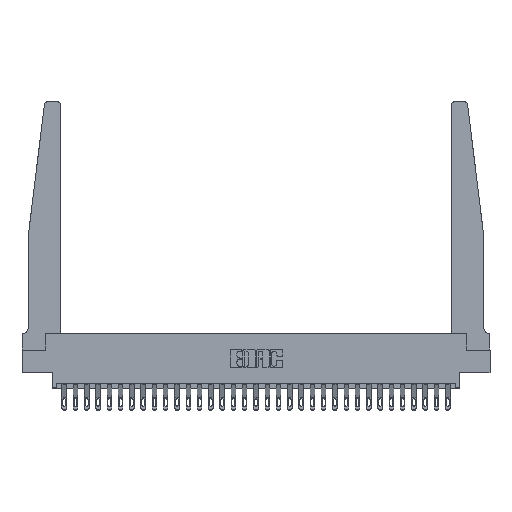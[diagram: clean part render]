
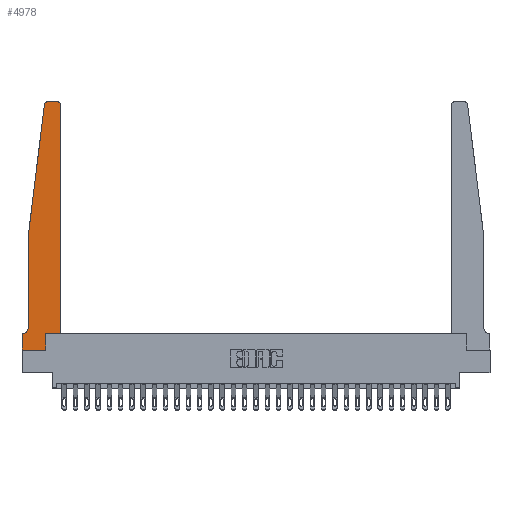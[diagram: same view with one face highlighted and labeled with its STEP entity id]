
A CAD part, top view. The second image highlights one B-rep face of the part: STEP entity #4978.
In plain terms, the highlighted planar face has unit normal (0, 0, 1).
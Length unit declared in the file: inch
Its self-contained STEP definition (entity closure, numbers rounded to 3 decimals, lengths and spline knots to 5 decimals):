
#320 = DIRECTION ( 'NONE',  ( 1., 0., 0. ) ) ;
#782 = VECTOR ( 'NONE', #8083, 39.37008 ) ;
#801 = VECTOR ( 'NONE', #20640, 39.37008 ) ;
#812 = CARTESIAN_POINT ( 'NONE',  ( 0.425, 0.18, 0.37 ) ) ;
#824 = AXIS2_PLACEMENT_3D ( 'NONE', #27190, #13727, #320 ) ;
#2477 = EDGE_CURVE ( 'NONE', #11949, #20682, #16619, .T. ) ;
#2863 = VERTEX_POINT ( 'NONE', #5621 ) ;
#3533 = CARTESIAN_POINT ( 'NONE',  ( 0.27653, 2.75, 0.37 ) ) ;
#3816 = EDGE_CURVE ( 'NONE', #6763, #6509, #17950, .T. ) ;
#3834 = VERTEX_POINT ( 'NONE', #5070 ) ;
#4319 = CARTESIAN_POINT ( 'NONE',  ( 0.2605, 0., 0.37 ) ) ;
#4370 = CARTESIAN_POINT ( 'NONE',  ( 0.395, 2.75, 0.37 ) ) ;
#4636 = DIRECTION ( 'NONE',  ( 0., 0., -1. ) ) ;
#4846 = CARTESIAN_POINT ( 'NONE',  ( 0., 0.1875, 0.37 ) ) ;
#4978 = ADVANCED_FACE ( 'NONE', ( #24131 ), #9467, .T. ) ;
#5057 = EDGE_CURVE ( 'NONE', #20908, #8378, #22018, .T. ) ;
#5070 = CARTESIAN_POINT ( 'NONE',  ( 0.015, 0.1875, 0.37 ) ) ;
#5209 = CIRCLE ( 'NONE', #824, 0.03 ) ;
#5621 = CARTESIAN_POINT ( 'NONE',  ( 0.425, 0.18, 0.37 ) ) ;
#6509 = VERTEX_POINT ( 'NONE', #3533 ) ;
#6750 = LINE ( 'NONE', #12464, #782 ) ;
#6763 = VERTEX_POINT ( 'NONE', #4370 ) ;
#7297 = ORIENTED_EDGE ( 'NONE', *, *, #3816, .T. ) ;
#7327 = DIRECTION ( 'NONE',  ( 1., 0., 0. ) ) ;
#7530 = CARTESIAN_POINT ( 'NONE',  ( 0., 0., 0.37 ) ) ;
#7535 = DIRECTION ( 'NONE',  ( 0., -1., 0. ) ) ;
#7594 = ORIENTED_EDGE ( 'NONE', *, *, #27460, .T. ) ;
#7862 = VERTEX_POINT ( 'NONE', #24970 ) ;
#7977 = VECTOR ( 'NONE', #26156, 39.37008 ) ;
#8083 = DIRECTION ( 'NONE',  ( -0.122, -0.992, 0. ) ) ;
#8378 = VERTEX_POINT ( 'NONE', #18049 ) ;
#8892 = ORIENTED_EDGE ( 'NONE', *, *, #24839, .T. ) ;
#9230 = ORIENTED_EDGE ( 'NONE', *, *, #19029, .T. ) ;
#9361 = VECTOR ( 'NONE', #14224, 39.37008 ) ;
#9467 = PLANE ( 'NONE',  #29012 ) ;
#10032 = CARTESIAN_POINT ( 'NONE',  ( 0.2605, 0.18, 0.37 ) ) ;
#10102 = VECTOR ( 'NONE', #7535, 39.37008 ) ;
#10426 = CARTESIAN_POINT ( 'NONE',  ( 0.395, 2.72, 0.37 ) ) ;
#10436 = CARTESIAN_POINT ( 'NONE',  ( 0., 0., 0.37 ) ) ;
#10691 = VECTOR ( 'NONE', #20111, 39.37008 ) ;
#10889 = CARTESIAN_POINT ( 'NONE',  ( 0.065, 1.25, 0.37 ) ) ;
#11316 = EDGE_CURVE ( 'NONE', #8378, #3834, #21455, .T. ) ;
#11502 = AXIS2_PLACEMENT_3D ( 'NONE', #10426, #26145, #12683 ) ;
#11662 = LINE ( 'NONE', #11758, #28841 ) ;
#11714 = DIRECTION ( 'NONE',  ( 0., 0., 1. ) ) ;
#11734 = CARTESIAN_POINT ( 'NONE',  ( 0.25, 2.75, 0.37 ) ) ;
#11758 = CARTESIAN_POINT ( 'NONE',  ( 0.065, 0.1875, 0.37 ) ) ;
#11949 = VERTEX_POINT ( 'NONE', #4319 ) ;
#12272 = ORIENTED_EDGE ( 'NONE', *, *, #5057, .T. ) ;
#12464 = CARTESIAN_POINT ( 'NONE',  ( 0.065, 1.25, 0.37 ) ) ;
#12683 = DIRECTION ( 'NONE',  ( 1., 0., 0. ) ) ;
#13025 = EDGE_CURVE ( 'NONE', #7862, #6763, #26985, .T. ) ;
#13501 = VERTEX_POINT ( 'NONE', #16437 ) ;
#13502 = EDGE_CURVE ( 'NONE', #2863, #7862, #25973, .T. ) ;
#13727 = DIRECTION ( 'NONE',  ( 0., 0., 1. ) ) ;
#13865 = AXIS2_PLACEMENT_3D ( 'NONE', #18037, #4636, #20295 ) ;
#14085 = EDGE_CURVE ( 'NONE', #6509, #24992, #5209, .T. ) ;
#14224 = DIRECTION ( 'NONE',  ( 0., -1., 0. ) ) ;
#14354 = EDGE_LOOP ( 'NONE', ( #7297, #20158, #7594, #12272, #16074, #26431, #9230, #8892, #23126, #25902, #26810, #16921 ) ) ;
#15273 = LINE ( 'NONE', #7530, #9361 ) ;
#15291 = CARTESIAN_POINT ( 'NONE',  ( 0.24675, 2.72367, 0.37 ) ) ;
#16074 = ORIENTED_EDGE ( 'NONE', *, *, #11316, .T. ) ;
#16437 = CARTESIAN_POINT ( 'NONE',  ( 0., 0.1875, 0.37 ) ) ;
#16619 = LINE ( 'NONE', #17858, #10691 ) ;
#16921 = ORIENTED_EDGE ( 'NONE', *, *, #13025, .T. ) ;
#17034 = EDGE_CURVE ( 'NONE', #20682, #2863, #26119, .T. ) ;
#17858 = CARTESIAN_POINT ( 'NONE',  ( 0.2605, 0.18, 0.37 ) ) ;
#17950 = LINE ( 'NONE', #11734, #801 ) ;
#18037 = CARTESIAN_POINT ( 'NONE',  ( 0.015, 0.2375, 0.37 ) ) ;
#18049 = CARTESIAN_POINT ( 'NONE',  ( 0.065, 0.2375, 0.37 ) ) ;
#19029 = EDGE_CURVE ( 'NONE', #13501, #23873, #15273, .T. ) ;
#19403 = VECTOR ( 'NONE', #7327, 39.37008 ) ;
#20111 = DIRECTION ( 'NONE',  ( 0., 1., 0. ) ) ;
#20158 = ORIENTED_EDGE ( 'NONE', *, *, #14085, .T. ) ;
#20295 = DIRECTION ( 'NONE',  ( -1., 0., 0. ) ) ;
#20640 = DIRECTION ( 'NONE',  ( -1., 0., 0. ) ) ;
#20682 = VERTEX_POINT ( 'NONE', #10032 ) ;
#20716 = CARTESIAN_POINT ( 'NONE',  ( 0.425, 0.18, 0.37 ) ) ;
#20908 = VERTEX_POINT ( 'NONE', #10889 ) ;
#21181 = EDGE_CURVE ( 'NONE', #3834, #13501, #11662, .T. ) ;
#21455 = CIRCLE ( 'NONE', #13865, 0.05 ) ;
#22018 = LINE ( 'NONE', #23186, #10102 ) ;
#23018 = LINE ( 'NONE', #10436, #7977 ) ;
#23037 = DIRECTION ( 'NONE',  ( -1., 0., 0. ) ) ;
#23126 = ORIENTED_EDGE ( 'NONE', *, *, #2477, .T. ) ;
#23186 = CARTESIAN_POINT ( 'NONE',  ( 0.065, 1.25, 0.37 ) ) ;
#23873 = VERTEX_POINT ( 'NONE', #26577 ) ;
#24131 = FACE_OUTER_BOUND ( 'NONE', #14354, .T. ) ;
#24839 = EDGE_CURVE ( 'NONE', #23873, #11949, #23018, .T. ) ;
#24970 = CARTESIAN_POINT ( 'NONE',  ( 0.425, 2.72, 0.37 ) ) ;
#24992 = VERTEX_POINT ( 'NONE', #15291 ) ;
#25245 = VECTOR ( 'NONE', #25517, 39.37008 ) ;
#25517 = DIRECTION ( 'NONE',  ( 0., 1., 0. ) ) ;
#25902 = ORIENTED_EDGE ( 'NONE', *, *, #17034, .T. ) ;
#25973 = LINE ( 'NONE', #812, #25245 ) ;
#26119 = LINE ( 'NONE', #20716, #19403 ) ;
#26145 = DIRECTION ( 'NONE',  ( 0., 0., 1. ) ) ;
#26156 = DIRECTION ( 'NONE',  ( 1., 0., 0. ) ) ;
#26431 = ORIENTED_EDGE ( 'NONE', *, *, #21181, .T. ) ;
#26577 = CARTESIAN_POINT ( 'NONE',  ( 0., 0., 0.37 ) ) ;
#26810 = ORIENTED_EDGE ( 'NONE', *, *, #13502, .T. ) ;
#26985 = CIRCLE ( 'NONE', #11502, 0.03 ) ;
#27190 = CARTESIAN_POINT ( 'NONE',  ( 0.27653, 2.72, 0.37 ) ) ;
#27402 = DIRECTION ( 'NONE',  ( 1., 0., 0. ) ) ;
#27460 = EDGE_CURVE ( 'NONE', #24992, #20908, #6750, .T. ) ;
#28841 = VECTOR ( 'NONE', #23037, 39.37008 ) ;
#29012 = AXIS2_PLACEMENT_3D ( 'NONE', #4846, #11714, #27402 ) ;
